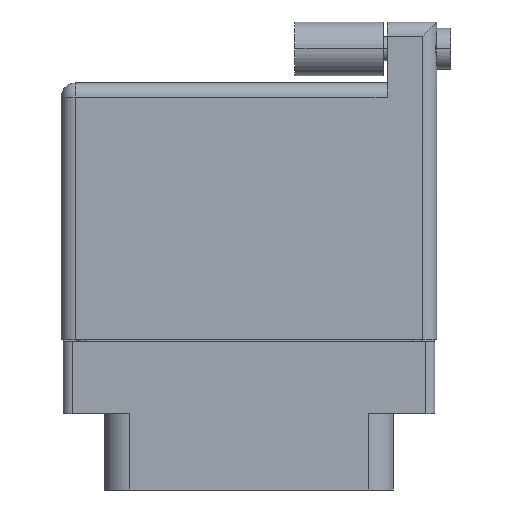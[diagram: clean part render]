
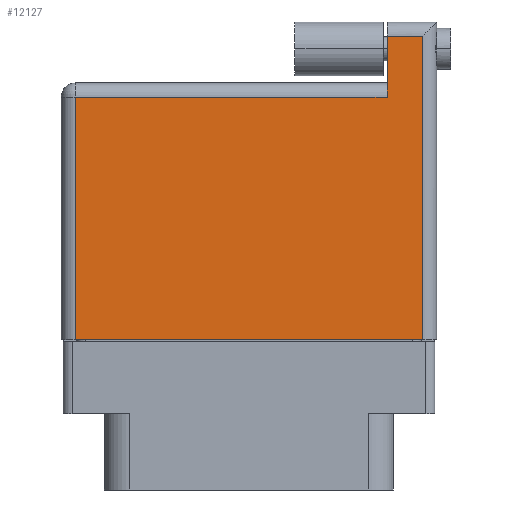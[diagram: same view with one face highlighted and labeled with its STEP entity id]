
A CAD part, front view. The second image highlights one B-rep face of the part: STEP entity #12127.
In plain terms, the highlighted face is planar.
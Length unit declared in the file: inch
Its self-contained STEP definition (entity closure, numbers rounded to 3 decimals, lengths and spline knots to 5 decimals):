
#163 = EDGE_CURVE ( 'NONE', #23749, #15514, #25947, .T. ) ;
#216 = LINE ( 'NONE', #17098, #17541 ) ;
#1301 = VECTOR ( 'NONE', #3161, 39.37008 ) ;
#1467 = ORIENTED_EDGE ( 'NONE', *, *, #10859, .T. ) ;
#1510 = EDGE_CURVE ( 'NONE', #15514, #8899, #24648, .T. ) ;
#1894 = EDGE_CURVE ( 'NONE', #2104, #8510, #11044, .T. ) ;
#2104 = VERTEX_POINT ( 'NONE', #15863 ) ;
#3161 = DIRECTION ( 'NONE',  ( -1., 0., 0. ) ) ;
#6022 = CARTESIAN_POINT ( 'NONE',  ( -0.6625, 0.756, 0.3575 ) ) ;
#6244 = EDGE_CURVE ( 'NONE', #8510, #23749, #16402, .T. ) ;
#7816 = DIRECTION ( 'NONE',  ( 0., 0., -1. ) ) ;
#7902 = ORIENTED_EDGE ( 'NONE', *, *, #1510, .T. ) ;
#8297 = DIRECTION ( 'NONE',  ( 1., 0., 0. ) ) ;
#8510 = VERTEX_POINT ( 'NONE', #13196 ) ;
#8899 = VERTEX_POINT ( 'NONE', #12477 ) ;
#9427 = DIRECTION ( 'NONE',  ( -1., 0., 0. ) ) ;
#9730 = CARTESIAN_POINT ( 'NONE',  ( -0.6625, 0.806, 0.3575 ) ) ;
#10300 = CARTESIAN_POINT ( 'NONE',  ( -0.6625, -0.1, 0.3575 ) ) ;
#10844 = ORIENTED_EDGE ( 'NONE', *, *, #24475, .T. ) ;
#10859 = EDGE_CURVE ( 'NONE', #19185, #2104, #23762, .T. ) ;
#11044 = LINE ( 'NONE', #20622, #21152 ) ;
#11686 = EDGE_LOOP ( 'NONE', ( #25144, #15437, #7902, #10844, #1467, #24008 ) ) ;
#12127 = ADVANCED_FACE ( 'NONE', ( #25286 ), #19791, .F. ) ;
#12173 = AXIS2_PLACEMENT_3D ( 'NONE', #9730, #7816, #23951 ) ;
#12477 = CARTESIAN_POINT ( 'NONE',  ( 0.4875, 0.97, 0.3575 ) ) ;
#13196 = CARTESIAN_POINT ( 'NONE',  ( -0.6125, -0.1, 0.3575 ) ) ;
#13253 = CARTESIAN_POINT ( 'NONE',  ( -0.6625, 0.97, 0.3575 ) ) ;
#14135 = CARTESIAN_POINT ( 'NONE',  ( 0.4875, 0.756, 0.3575 ) ) ;
#14812 = DIRECTION ( 'NONE',  ( 0., -1., 0. ) ) ;
#15437 = ORIENTED_EDGE ( 'NONE', *, *, #163, .T. ) ;
#15514 = VERTEX_POINT ( 'NONE', #17832 ) ;
#15823 = CARTESIAN_POINT ( 'NONE',  ( 0.6125, 1.02, 0.3575 ) ) ;
#15863 = CARTESIAN_POINT ( 'NONE',  ( -0.6125, 0.756, 0.3575 ) ) ;
#16402 = LINE ( 'NONE', #10300, #18303 ) ;
#17098 = CARTESIAN_POINT ( 'NONE',  ( 0.4875, 1.02, 0.3575 ) ) ;
#17541 = VECTOR ( 'NONE', #23184, 39.37008 ) ;
#17832 = CARTESIAN_POINT ( 'NONE',  ( 0.6125, 0.97, 0.3575 ) ) ;
#17844 = DIRECTION ( 'NONE',  ( 0., 1., 0. ) ) ;
#18303 = VECTOR ( 'NONE', #8297, 39.37008 ) ;
#19185 = VERTEX_POINT ( 'NONE', #14135 ) ;
#19791 = PLANE ( 'NONE',  #12173 ) ;
#20622 = CARTESIAN_POINT ( 'NONE',  ( -0.6125, -0.1, 0.3575 ) ) ;
#21152 = VECTOR ( 'NONE', #14812, 39.37008 ) ;
#23130 = VECTOR ( 'NONE', #9427, 39.37008 ) ;
#23184 = DIRECTION ( 'NONE',  ( 0., -1., 0. ) ) ;
#23749 = VERTEX_POINT ( 'NONE', #24806 ) ;
#23762 = LINE ( 'NONE', #6022, #23130 ) ;
#23951 = DIRECTION ( 'NONE',  ( -1., 0., 0. ) ) ;
#24008 = ORIENTED_EDGE ( 'NONE', *, *, #1894, .T. ) ;
#24475 = EDGE_CURVE ( 'NONE', #8899, #19185, #216, .T. ) ;
#24648 = LINE ( 'NONE', #13253, #1301 ) ;
#24689 = VECTOR ( 'NONE', #17844, 39.37008 ) ;
#24806 = CARTESIAN_POINT ( 'NONE',  ( 0.6125, -0.1, 0.3575 ) ) ;
#25144 = ORIENTED_EDGE ( 'NONE', *, *, #6244, .T. ) ;
#25286 = FACE_OUTER_BOUND ( 'NONE', #11686, .T. ) ;
#25947 = LINE ( 'NONE', #15823, #24689 ) ;
